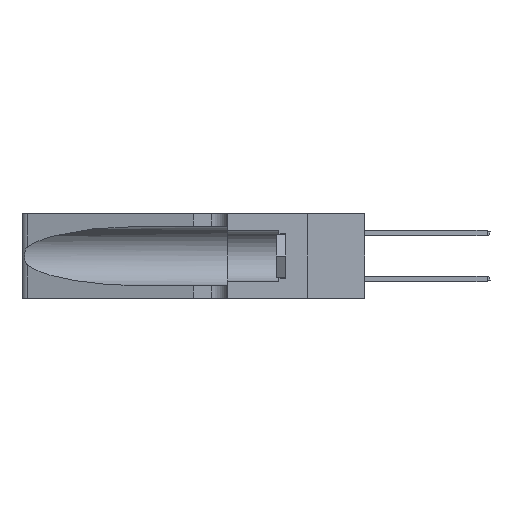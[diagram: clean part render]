
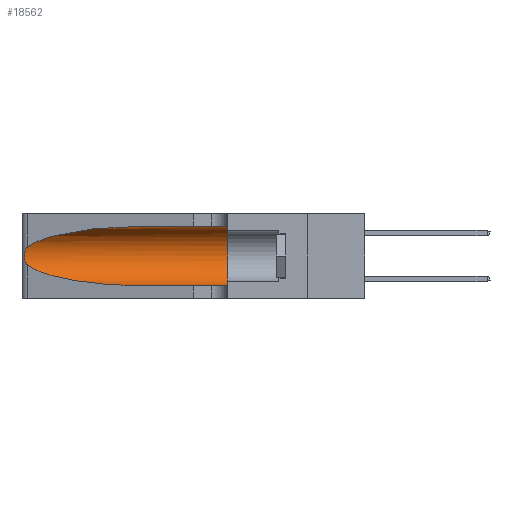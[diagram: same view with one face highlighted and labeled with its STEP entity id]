
A CAD part, left-side view. The second image highlights one B-rep face of the part: STEP entity #18562.
In plain terms, the highlighted cylindrical face has radius 3.308 mm (diameter 6.617 mm), a partial arc.
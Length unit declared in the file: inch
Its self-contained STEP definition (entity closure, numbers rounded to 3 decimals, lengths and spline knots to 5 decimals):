
#655 = EDGE_CURVE ( 'NONE', #37397, #17371, #2396, .T. ) ;
#1316 = VERTEX_POINT ( 'NONE', #2016 ) ;
#1876 = DIRECTION ( 'NONE',  ( 0., -1., 0. ) ) ;
#2016 = CARTESIAN_POINT ( 'NONE',  ( 0.25487, 1.22718, 0.14631 ) ) ;
#2396 =( BOUNDED_CURVE ( )  B_SPLINE_CURVE ( 3, ( #20068, #20143, #20565, #19709 ),
 .UNSPECIFIED., .F., .T. ) 
 B_SPLINE_CURVE_WITH_KNOTS ( ( 4, 4 ),
 ( 1.5708, 2.84003 ),
 .UNSPECIFIED. ) 
 CURVE ( )  GEOMETRIC_REPRESENTATION_ITEM ( )  RATIONAL_B_SPLINE_CURVE ( ( 1., 0.87, 0.87, 1. ) ) 
 REPRESENTATION_ITEM ( '' )  );
#4075 = CARTESIAN_POINT ( 'NONE',  ( 0.25487, 1.22718, 0.22369 ) ) ;
#4208 = CARTESIAN_POINT ( 'NONE',  ( 0.25787, 1.23484, 0.2124 ) ) ;
#6258 = CARTESIAN_POINT ( 'NONE',  ( 0.1305, 1.61858, 0.31525 ) ) ;
#6698 = CARTESIAN_POINT ( 'NONE',  ( 0.2373, 1.15595, 0.08982 ) ) ;
#6759 = EDGE_CURVE ( 'NONE', #1316, #7348, #33570, .T. ) ;
#7194 = CARTESIAN_POINT ( 'NONE',  ( 0.26018, 1.23835, 0.19895 ) ) ;
#7348 = VERTEX_POINT ( 'NONE', #18055 ) ;
#8803 = ORIENTED_EDGE ( 'NONE', *, *, #6759, .T. ) ;
#9653 = CARTESIAN_POINT ( 'NONE',  ( 0.25487, 1.22718, 0.14631 ) ) ;
#9742 = CYLINDRICAL_SURFACE ( 'NONE', #31270, 0.13025 ) ;
#10021 = VERTEX_POINT ( 'NONE', #23055 ) ;
#10150 = CARTESIAN_POINT ( 'NONE',  ( 0.26075, 1.23896, 0.178 ) ) ;
#11788 = LINE ( 'NONE', #33672, #34105 ) ;
#12163 = ORIENTED_EDGE ( 'NONE', *, *, #23475, .F. ) ;
#13108 = CARTESIAN_POINT ( 'NONE',  ( 0.25856, 1.23593, 0.16098 ) ) ;
#14394 = DIRECTION ( 'NONE',  ( 0., 1., 0. ) ) ;
#14531 = AXIS2_PLACEMENT_3D ( 'NONE', #31843, #14394, #34734 ) ;
#15500 = CIRCLE ( 'NONE', #14531, 0.13025 ) ;
#15539 = CARTESIAN_POINT ( 'NONE',  ( 0.1305, 0.72297, 0.05475 ) ) ;
#15763 = EDGE_LOOP ( 'NONE', ( #18014, #36949, #8803, #32431, #12163, #19203 ) ) ;
#16032 = CARTESIAN_POINT ( 'NONE',  ( 0.25639, 1.23186, 0.15144 ) ) ;
#16568 = CARTESIAN_POINT ( 'NONE',  ( 0.1305, 1.61858, 0.185 ) ) ;
#17371 = VERTEX_POINT ( 'NONE', #34686 ) ;
#18014 = ORIENTED_EDGE ( 'NONE', *, *, #655, .T. ) ;
#18055 = CARTESIAN_POINT ( 'NONE',  ( 0.1305, 0.72297, 0.05475 ) ) ;
#18562 = ADVANCED_FACE ( 'NONE', ( #20240 ), #9742, .F. ) ;
#18982 = CARTESIAN_POINT ( 'NONE',  ( 0.25487, 1.22718, 0.14631 ) ) ;
#19203 = ORIENTED_EDGE ( 'NONE', *, *, #27392, .F. ) ;
#19493 = DIRECTION ( 'NONE',  ( 0., 0., -1. ) ) ;
#19709 = CARTESIAN_POINT ( 'NONE',  ( 0.25487, 1.22718, 0.22369 ) ) ;
#20068 = CARTESIAN_POINT ( 'NONE',  ( 0.1305, 0.72297, 0.31525 ) ) ;
#20143 = CARTESIAN_POINT ( 'NONE',  ( 0.18966, 0.96281, 0.31525 ) ) ;
#20240 = FACE_OUTER_BOUND ( 'NONE', #15763, .T. ) ;
#20290 = CARTESIAN_POINT ( 'NONE',  ( 0.1305, 0.35, 0.05475 ) ) ;
#20565 = CARTESIAN_POINT ( 'NONE',  ( 0.2373, 1.15595, 0.28018 ) ) ;
#21734 = CARTESIAN_POINT ( 'NONE',  ( 0.25639, 1.23184, 0.21858 ) ) ;
#23055 = CARTESIAN_POINT ( 'NONE',  ( 0.1305, 0.35, 0.31525 ) ) ;
#23475 = EDGE_CURVE ( 'NONE', #10021, #27956, #15500, .T. ) ;
#24639 = CARTESIAN_POINT ( 'NONE',  ( 0.25854, 1.2359, 0.20912 ) ) ;
#24713 = VECTOR ( 'NONE', #26562, 39.37008 ) ;
#26562 = DIRECTION ( 'NONE',  ( 0., -1., 0. ) ) ;
#27392 = EDGE_CURVE ( 'NONE', #37397, #10021, #33412, .T. ) ;
#27597 = CARTESIAN_POINT ( 'NONE',  ( 0.26075, 1.23896, 0.19203 ) ) ;
#27956 = VERTEX_POINT ( 'NONE', #20290 ) ;
#30541 = CARTESIAN_POINT ( 'NONE',  ( 0.26017, 1.23833, 0.17102 ) ) ;
#31270 = AXIS2_PLACEMENT_3D ( 'NONE', #16568, #1876, #19493 ) ;
#31843 = CARTESIAN_POINT ( 'NONE',  ( 0.1305, 0.35, 0.185 ) ) ;
#32431 = ORIENTED_EDGE ( 'NONE', *, *, #33539, .T. ) ;
#32825 = EDGE_CURVE ( 'NONE', #17371, #1316, #34718, .T. ) ;
#32974 = CARTESIAN_POINT ( 'NONE',  ( 0.18966, 0.96281, 0.05475 ) ) ;
#33336 = CARTESIAN_POINT ( 'NONE',  ( 0.25555, 1.22994, 0.2215 ) ) ;
#33412 = LINE ( 'NONE', #6258, #24713 ) ;
#33464 = CARTESIAN_POINT ( 'NONE',  ( 0.25789, 1.23486, 0.15765 ) ) ;
#33539 = EDGE_CURVE ( 'NONE', #7348, #27956, #11788, .T. ) ;
#33570 =( BOUNDED_CURVE ( )  B_SPLINE_CURVE ( 3, ( #9653, #6698, #32974, #15539 ),
 .UNSPECIFIED., .F., .F. ) 
 B_SPLINE_CURVE_WITH_KNOTS ( ( 4, 4 ),
 ( 3.44316, 4.71239 ),
 .UNSPECIFIED. ) 
 CURVE ( )  GEOMETRIC_REPRESENTATION_ITEM ( )  RATIONAL_B_SPLINE_CURVE ( ( 1., 0.87, 0.87, 1. ) ) 
 REPRESENTATION_ITEM ( '' )  );
#33672 = CARTESIAN_POINT ( 'NONE',  ( 0.1305, 1.61858, 0.05475 ) ) ;
#34105 = VECTOR ( 'NONE', #36544, 39.37008 ) ;
#34686 = CARTESIAN_POINT ( 'NONE',  ( 0.25487, 1.22718, 0.22369 ) ) ;
#34718 = B_SPLINE_CURVE_WITH_KNOTS ( 'NONE', 3,
 ( #4075, #33336, #21734, #4208, #24639, #7194, #27597, #10150, #30541, #13108, #33464, #16032, #36345, #18982 ),
 .UNSPECIFIED., .F., .F.,
 ( 4, 2, 2, 2, 2, 2, 4 ),
 ( 0., 0.00027, 0.00053, 0.00107, 0.0016, 0.00187, 0.00214 ),
 .UNSPECIFIED. ) ;
#34734 = DIRECTION ( 'NONE',  ( 0., 0., 1. ) ) ;
#36345 = CARTESIAN_POINT ( 'NONE',  ( 0.25555, 1.22993, 0.14849 ) ) ;
#36544 = DIRECTION ( 'NONE',  ( 0., -1., 0. ) ) ;
#36949 = ORIENTED_EDGE ( 'NONE', *, *, #32825, .T. ) ;
#37397 = VERTEX_POINT ( 'NONE', #37424 ) ;
#37424 = CARTESIAN_POINT ( 'NONE',  ( 0.1305, 0.72297, 0.31525 ) ) ;
